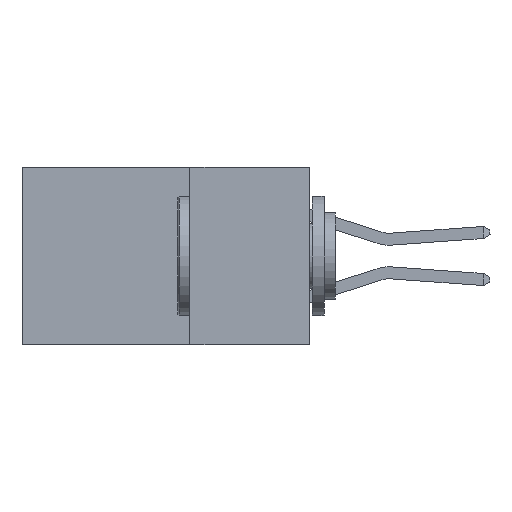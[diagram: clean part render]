
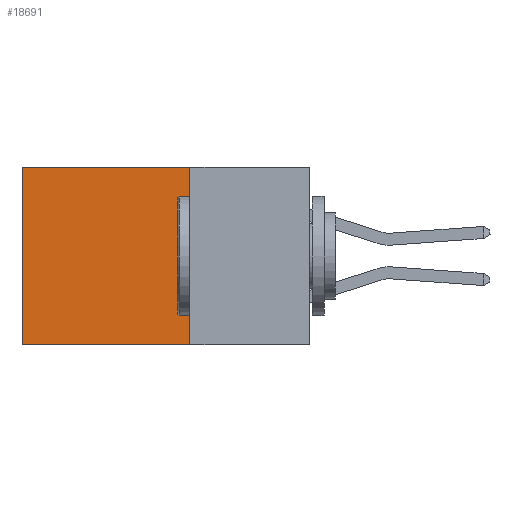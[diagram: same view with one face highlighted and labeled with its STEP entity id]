
A CAD part, left-side view. The second image highlights one B-rep face of the part: STEP entity #18691.
In plain terms, the highlighted planar face has unit normal (-1, 0, 0).
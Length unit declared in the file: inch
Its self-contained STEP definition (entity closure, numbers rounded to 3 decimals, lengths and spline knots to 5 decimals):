
#577 = PLANE ( 'NONE',  #2069 ) ;
#946 = ORIENTED_EDGE ( 'NONE', *, *, #14464, .F. ) ;
#2069 = AXIS2_PLACEMENT_3D ( 'NONE', #25819, #2714, #17470 ) ;
#2118 = EDGE_LOOP ( 'NONE', ( #10518, #7719, #946, #3200 ) ) ;
#2572 = EDGE_CURVE ( 'NONE', #6130, #7137, #9395, .T. ) ;
#2714 = DIRECTION ( 'NONE',  ( 1., 0., 0. ) ) ;
#3200 = ORIENTED_EDGE ( 'NONE', *, *, #13609, .T. ) ;
#3719 = VERTEX_POINT ( 'NONE', #22390 ) ;
#3756 = VECTOR ( 'NONE', #11679, 39.37008 ) ;
#4152 = LINE ( 'NONE', #8208, #14691 ) ;
#6117 = DIRECTION ( 'NONE',  ( 0., 1., 0. ) ) ;
#6130 = VERTEX_POINT ( 'NONE', #19176 ) ;
#7137 = VERTEX_POINT ( 'NONE', #11831 ) ;
#7356 = DIRECTION ( 'NONE',  ( 0., 0., -1. ) ) ;
#7719 = ORIENTED_EDGE ( 'NONE', *, *, #22330, .F. ) ;
#8208 = CARTESIAN_POINT ( 'NONE',  ( 0.2615, 0.25, -0.37 ) ) ;
#8446 = CARTESIAN_POINT ( 'NONE',  ( 0.2615, 0.25, -0.37 ) ) ;
#8990 = CARTESIAN_POINT ( 'NONE',  ( 0.2615, 0.6, -0.37 ) ) ;
#9395 = LINE ( 'NONE', #8990, #18674 ) ;
#9552 = CARTESIAN_POINT ( 'NONE',  ( 0.2615, 0.25, 0. ) ) ;
#10021 = LINE ( 'NONE', #9552, #3756 ) ;
#10518 = ORIENTED_EDGE ( 'NONE', *, *, #2572, .T. ) ;
#11074 = VERTEX_POINT ( 'NONE', #26632 ) ;
#11679 = DIRECTION ( 'NONE',  ( 0., 1., 0. ) ) ;
#11831 = CARTESIAN_POINT ( 'NONE',  ( 0.2615, 0.6, -0.37 ) ) ;
#13609 = EDGE_CURVE ( 'NONE', #3719, #6130, #10021, .T. ) ;
#14464 = EDGE_CURVE ( 'NONE', #3719, #11074, #16616, .T. ) ;
#14691 = VECTOR ( 'NONE', #6117, 39.37008 ) ;
#16616 = LINE ( 'NONE', #8446, #22903 ) ;
#17470 = DIRECTION ( 'NONE',  ( 0., 0., -1. ) ) ;
#18674 = VECTOR ( 'NONE', #7356, 39.37008 ) ;
#18691 = ADVANCED_FACE ( 'NONE', ( #20544 ), #577, .F. ) ;
#19176 = CARTESIAN_POINT ( 'NONE',  ( 0.2615, 0.6, 0. ) ) ;
#20544 = FACE_OUTER_BOUND ( 'NONE', #2118, .T. ) ;
#22330 = EDGE_CURVE ( 'NONE', #11074, #7137, #4152, .T. ) ;
#22390 = CARTESIAN_POINT ( 'NONE',  ( 0.2615, 0.25, 0. ) ) ;
#22903 = VECTOR ( 'NONE', #23230, 39.37008 ) ;
#23230 = DIRECTION ( 'NONE',  ( 0., 0., -1. ) ) ;
#25819 = CARTESIAN_POINT ( 'NONE',  ( 0.2615, 0.25, -0.37 ) ) ;
#26632 = CARTESIAN_POINT ( 'NONE',  ( 0.2615, 0.25, -0.37 ) ) ;
